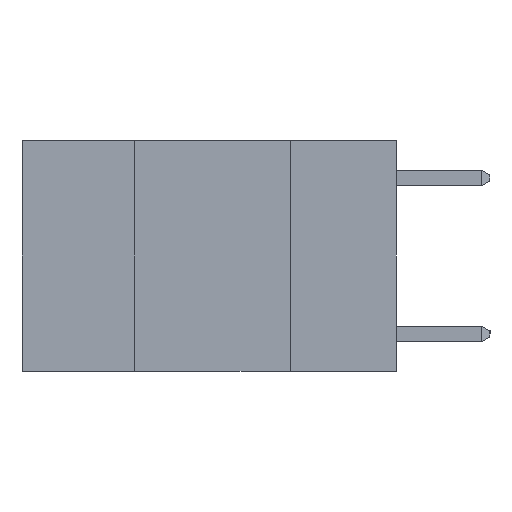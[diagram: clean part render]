
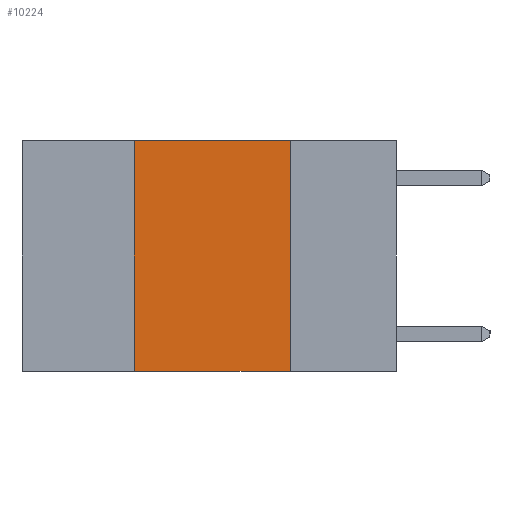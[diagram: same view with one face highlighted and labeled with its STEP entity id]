
A CAD part, left-side view. The second image highlights one B-rep face of the part: STEP entity #10224.
In plain terms, the highlighted planar face has unit normal (-1, 0, 0).
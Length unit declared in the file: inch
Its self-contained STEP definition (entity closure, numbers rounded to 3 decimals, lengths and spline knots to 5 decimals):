
#178 = EDGE_CURVE ( 'NONE', #7110, #6329, #4951, .T. ) ;
#1121 = VERTEX_POINT ( 'NONE', #3735 ) ;
#1656 = ORIENTED_EDGE ( 'NONE', *, *, #7812, .F. ) ;
#1877 = PLANE ( 'NONE',  #3288 ) ;
#1891 = ORIENTED_EDGE ( 'NONE', *, *, #3489, .T. ) ;
#2901 = LINE ( 'NONE', #4302, #7955 ) ;
#3015 = DIRECTION ( 'NONE',  ( 1., 0., 0. ) ) ;
#3068 = DIRECTION ( 'NONE',  ( 0., 0., -1. ) ) ;
#3288 = AXIS2_PLACEMENT_3D ( 'NONE', #9520, #3015, #9559 ) ;
#3411 = EDGE_CURVE ( 'NONE', #1121, #6285, #6414, .T. ) ;
#3489 = EDGE_CURVE ( 'NONE', #1121, #6329, #2901, .T. ) ;
#3735 = CARTESIAN_POINT ( 'NONE',  ( 0., 0.42, -0.37 ) ) ;
#3885 = VECTOR ( 'NONE', #5149, 39.37008 ) ;
#4124 = CARTESIAN_POINT ( 'NONE',  ( 0., 0.42, 0. ) ) ;
#4125 = ORIENTED_EDGE ( 'NONE', *, *, #178, .F. ) ;
#4259 = DIRECTION ( 'NONE',  ( 0., -1., 0. ) ) ;
#4302 = CARTESIAN_POINT ( 'NONE',  ( 0., 0.6, -0.37 ) ) ;
#4951 = LINE ( 'NONE', #9682, #7081 ) ;
#5149 = DIRECTION ( 'NONE',  ( 0., 0., 1. ) ) ;
#5278 = DIRECTION ( 'NONE',  ( 0., -1., 0. ) ) ;
#6285 = VERTEX_POINT ( 'NONE', #8981 ) ;
#6329 = VERTEX_POINT ( 'NONE', #11641 ) ;
#6414 = LINE ( 'NONE', #4124, #3885 ) ;
#6464 = FACE_OUTER_BOUND ( 'NONE', #6543, .T. ) ;
#6543 = EDGE_LOOP ( 'NONE', ( #4125, #1656, #7543, #1891 ) ) ;
#7081 = VECTOR ( 'NONE', #3068, 39.37008 ) ;
#7110 = VERTEX_POINT ( 'NONE', #9947 ) ;
#7543 = ORIENTED_EDGE ( 'NONE', *, *, #3411, .F. ) ;
#7779 = LINE ( 'NONE', #10620, #12216 ) ;
#7812 = EDGE_CURVE ( 'NONE', #6285, #7110, #7779, .T. ) ;
#7955 = VECTOR ( 'NONE', #5278, 39.37008 ) ;
#8981 = CARTESIAN_POINT ( 'NONE',  ( 0., 0.42, 0. ) ) ;
#9520 = CARTESIAN_POINT ( 'NONE',  ( 0., 0.6, 0. ) ) ;
#9559 = DIRECTION ( 'NONE',  ( 0., 0., -1. ) ) ;
#9682 = CARTESIAN_POINT ( 'NONE',  ( 0., 0.17, 0. ) ) ;
#9947 = CARTESIAN_POINT ( 'NONE',  ( 0., 0.17, 0. ) ) ;
#10224 = ADVANCED_FACE ( 'NONE', ( #6464 ), #1877, .F. ) ;
#10620 = CARTESIAN_POINT ( 'NONE',  ( 0., 0.6, 0. ) ) ;
#11641 = CARTESIAN_POINT ( 'NONE',  ( 0., 0.17, -0.37 ) ) ;
#12216 = VECTOR ( 'NONE', #4259, 39.37008 ) ;
